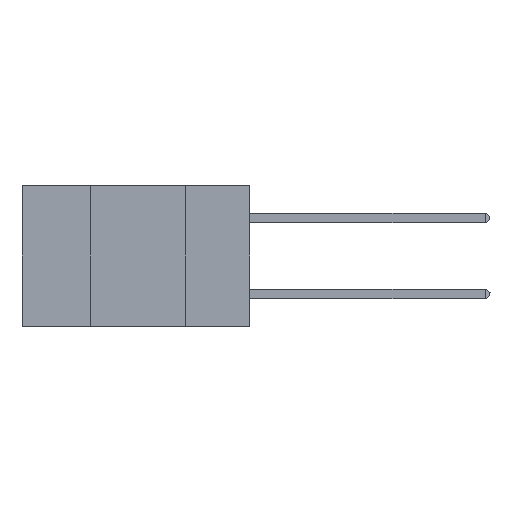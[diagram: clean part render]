
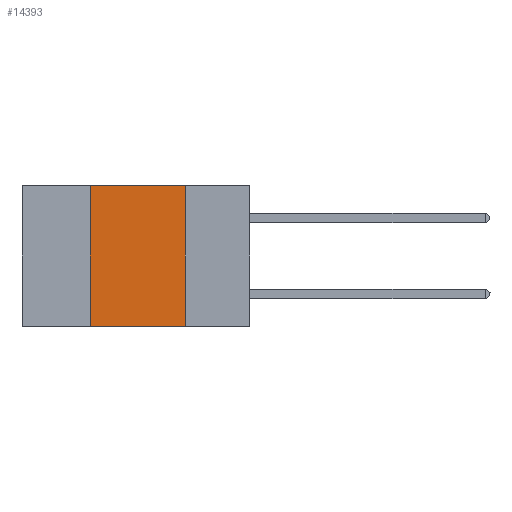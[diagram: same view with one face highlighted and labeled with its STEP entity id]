
A CAD part, left-side view. The second image highlights one B-rep face of the part: STEP entity #14393.
In plain terms, the highlighted planar face has unit normal (-1, 0, 0).
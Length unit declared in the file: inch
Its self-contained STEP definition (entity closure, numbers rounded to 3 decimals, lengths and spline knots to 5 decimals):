
#1154 = CARTESIAN_POINT ( 'NONE',  ( 0., 0.42, -0.37 ) ) ;
#1961 = DIRECTION ( 'NONE',  ( 0., 0., 1. ) ) ;
#2541 = ORIENTED_EDGE ( 'NONE', *, *, #19585, .T. ) ;
#3194 = PLANE ( 'NONE',  #27500 ) ;
#3434 = VERTEX_POINT ( 'NONE', #26922 ) ;
#5634 = VECTOR ( 'NONE', #26404, 39.37008 ) ;
#8245 = LINE ( 'NONE', #10713, #5634 ) ;
#8904 = ORIENTED_EDGE ( 'NONE', *, *, #10124, .F. ) ;
#10124 = EDGE_CURVE ( 'NONE', #21240, #3434, #28840, .T. ) ;
#10633 = EDGE_CURVE ( 'NONE', #13883, #21173, #13368, .T. ) ;
#10713 = CARTESIAN_POINT ( 'NONE',  ( 0., 0.6, -0.37 ) ) ;
#11333 = CARTESIAN_POINT ( 'NONE',  ( 0., 0.42, 0. ) ) ;
#12125 = DIRECTION ( 'NONE',  ( 0., 0., -1. ) ) ;
#12546 = CARTESIAN_POINT ( 'NONE',  ( 0., 0.6, 0. ) ) ;
#12809 = VECTOR ( 'NONE', #28136, 39.37008 ) ;
#13085 = DIRECTION ( 'NONE',  ( 0., 0., -1. ) ) ;
#13368 = LINE ( 'NONE', #28652, #15225 ) ;
#13883 = VERTEX_POINT ( 'NONE', #15826 ) ;
#14393 = ADVANCED_FACE ( 'NONE', ( #18714 ), #3194, .F. ) ;
#15225 = VECTOR ( 'NONE', #13085, 39.37008 ) ;
#15826 = CARTESIAN_POINT ( 'NONE',  ( 0., 0.17, 0. ) ) ;
#16498 = LINE ( 'NONE', #12546, #12809 ) ;
#18273 = DIRECTION ( 'NONE',  ( 1., 0., 0. ) ) ;
#18410 = CARTESIAN_POINT ( 'NONE',  ( 0., 0.6, 0. ) ) ;
#18714 = FACE_OUTER_BOUND ( 'NONE', #21835, .T. ) ;
#19585 = EDGE_CURVE ( 'NONE', #21240, #21173, #8245, .T. ) ;
#20959 = ORIENTED_EDGE ( 'NONE', *, *, #10633, .F. ) ;
#21173 = VERTEX_POINT ( 'NONE', #23582 ) ;
#21240 = VERTEX_POINT ( 'NONE', #1154 ) ;
#21835 = EDGE_LOOP ( 'NONE', ( #20959, #28182, #8904, #2541 ) ) ;
#23582 = CARTESIAN_POINT ( 'NONE',  ( 0., 0.17, -0.37 ) ) ;
#24099 = VECTOR ( 'NONE', #1961, 39.37008 ) ;
#24347 = EDGE_CURVE ( 'NONE', #3434, #13883, #16498, .T. ) ;
#26404 = DIRECTION ( 'NONE',  ( 0., -1., 0. ) ) ;
#26922 = CARTESIAN_POINT ( 'NONE',  ( 0., 0.42, 0. ) ) ;
#27500 = AXIS2_PLACEMENT_3D ( 'NONE', #18410, #18273, #12125 ) ;
#28136 = DIRECTION ( 'NONE',  ( 0., -1., 0. ) ) ;
#28182 = ORIENTED_EDGE ( 'NONE', *, *, #24347, .F. ) ;
#28652 = CARTESIAN_POINT ( 'NONE',  ( 0., 0.17, 0. ) ) ;
#28840 = LINE ( 'NONE', #11333, #24099 ) ;
